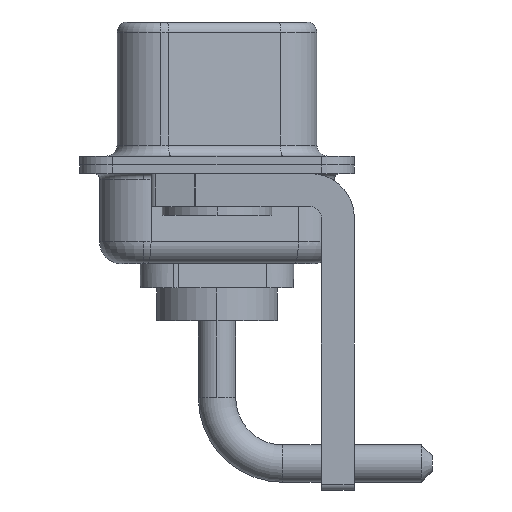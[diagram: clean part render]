
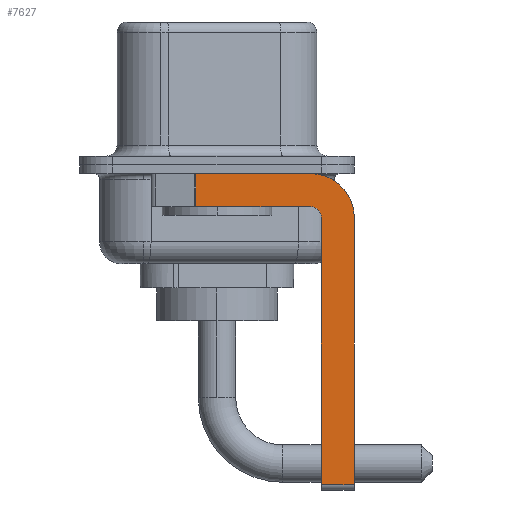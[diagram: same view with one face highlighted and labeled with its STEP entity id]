
A CAD part, left-side view. The second image highlights one B-rep face of the part: STEP entity #7627.
In plain terms, the highlighted planar face has unit normal (-1, 0, 0).
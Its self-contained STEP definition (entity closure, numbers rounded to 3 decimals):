
#83 = VECTOR ( 'NONE', #9557, 1000. ) ;
#357 = ORIENTED_EDGE ( 'NONE', *, *, #1026, .F. ) ;
#539 = VERTEX_POINT ( 'NONE', #1725 ) ;
#855 = CARTESIAN_POINT ( 'NONE',  ( -2.9, -4.25, -1.9 ) ) ;
#933 = LINE ( 'NONE', #855, #1453 ) ;
#1026 = EDGE_CURVE ( 'NONE', #9850, #12644, #933, .T. ) ;
#1371 = ORIENTED_EDGE ( 'NONE', *, *, #8969, .T. ) ;
#1448 = CARTESIAN_POINT ( 'NONE',  ( -2.9, -6.25, -2.4 ) ) ;
#1453 = VECTOR ( 'NONE', #13734, 1000. ) ;
#1725 = CARTESIAN_POINT ( 'NONE',  ( -2.9, 0.978, -0.4 ) ) ;
#1827 = DIRECTION ( 'NONE',  ( 0., -1., 0. ) ) ;
#2507 = ORIENTED_EDGE ( 'NONE', *, *, #12134, .F. ) ;
#3153 = CARTESIAN_POINT ( 'NONE',  ( -2.9, -4.25, -1.9 ) ) ;
#3434 = DIRECTION ( 'NONE',  ( 0., 0., 1. ) ) ;
#3773 = AXIS2_PLACEMENT_3D ( 'NONE', #8376, #5162, #3866 ) ;
#3866 = DIRECTION ( 'NONE',  ( 0., 0., -1. ) ) ;
#4071 = CARTESIAN_POINT ( 'NONE',  ( -2.9, -4.75, -2.4 ) ) ;
#4494 = ORIENTED_EDGE ( 'NONE', *, *, #10451, .F. ) ;
#4548 = VERTEX_POINT ( 'NONE', #13853 ) ;
#4583 = DIRECTION ( 'NONE',  ( -1., 0., 0. ) ) ;
#5088 = EDGE_CURVE ( 'NONE', #539, #12644, #9227, .T. ) ;
#5162 = DIRECTION ( 'NONE',  ( 1., 0., 0. ) ) ;
#5433 = EDGE_CURVE ( 'NONE', #11198, #10752, #10421, .T. ) ;
#5452 = CARTESIAN_POINT ( 'NONE',  ( -2.9, -4.75, -14.8 ) ) ;
#5649 = ORIENTED_EDGE ( 'NONE', *, *, #5433, .F. ) ;
#5971 = LINE ( 'NONE', #1448, #83 ) ;
#6918 = AXIS2_PLACEMENT_3D ( 'NONE', #12777, #4583, #3434 ) ;
#7002 = CARTESIAN_POINT ( 'NONE',  ( -2.9, -6.25, -2.4 ) ) ;
#7567 = PLANE ( 'NONE',  #11463 ) ;
#7627 = ADVANCED_FACE ( 'NONE', ( #12322 ), #7567, .F. ) ;
#7632 = LINE ( 'NONE', #13407, #8313 ) ;
#8090 = VECTOR ( 'NONE', #10533, 1000. ) ;
#8267 = VERTEX_POINT ( 'NONE', #7002 ) ;
#8292 = EDGE_LOOP ( 'NONE', ( #10989, #10676, #357, #4494, #5649, #1371, #12744, #2507 ) ) ;
#8313 = VECTOR ( 'NONE', #1827, 1000. ) ;
#8376 = CARTESIAN_POINT ( 'NONE',  ( -2.9, -4.25, -2.4 ) ) ;
#8795 = EDGE_CURVE ( 'NONE', #539, #11840, #7632, .T. ) ;
#8944 = CARTESIAN_POINT ( 'NONE',  ( -2.9, -4.75, -14.55 ) ) ;
#8969 = EDGE_CURVE ( 'NONE', #11198, #4548, #10297, .T. ) ;
#9178 = VECTOR ( 'NONE', #12586, 1000. ) ;
#9227 = LINE ( 'NONE', #13761, #14378 ) ;
#9557 = DIRECTION ( 'NONE',  ( 0., 0., -1. ) ) ;
#9850 = VERTEX_POINT ( 'NONE', #3153 ) ;
#10010 = DIRECTION ( 'NONE',  ( 0., 0., -1. ) ) ;
#10297 = LINE ( 'NONE', #13704, #8090 ) ;
#10360 = CIRCLE ( 'NONE', #3773, 2. ) ;
#10421 = LINE ( 'NONE', #5452, #9178 ) ;
#10451 = EDGE_CURVE ( 'NONE', #10752, #9850, #12793, .T. ) ;
#10533 = DIRECTION ( 'NONE',  ( 0., -1., 0. ) ) ;
#10676 = ORIENTED_EDGE ( 'NONE', *, *, #5088, .T. ) ;
#10752 = VERTEX_POINT ( 'NONE', #4071 ) ;
#10989 = ORIENTED_EDGE ( 'NONE', *, *, #8795, .F. ) ;
#11083 = EDGE_CURVE ( 'NONE', #8267, #4548, #5971, .T. ) ;
#11161 = CARTESIAN_POINT ( 'NONE',  ( -2.9, -4.25, -2.4 ) ) ;
#11198 = VERTEX_POINT ( 'NONE', #8944 ) ;
#11463 = AXIS2_PLACEMENT_3D ( 'NONE', #11161, #13559, #10010 ) ;
#11840 = VERTEX_POINT ( 'NONE', #15067 ) ;
#12134 = EDGE_CURVE ( 'NONE', #11840, #8267, #10360, .T. ) ;
#12322 = FACE_OUTER_BOUND ( 'NONE', #8292, .T. ) ;
#12401 = CARTESIAN_POINT ( 'NONE',  ( -2.9, 0.978, -1.9 ) ) ;
#12586 = DIRECTION ( 'NONE',  ( 0., 0., 1. ) ) ;
#12644 = VERTEX_POINT ( 'NONE', #12401 ) ;
#12744 = ORIENTED_EDGE ( 'NONE', *, *, #11083, .F. ) ;
#12777 = CARTESIAN_POINT ( 'NONE',  ( -2.9, -4.25, -2.4 ) ) ;
#12793 = CIRCLE ( 'NONE', #6918, 0.5 ) ;
#13407 = CARTESIAN_POINT ( 'NONE',  ( -2.9, 3., -0.4 ) ) ;
#13559 = DIRECTION ( 'NONE',  ( 1., 0., 0. ) ) ;
#13704 = CARTESIAN_POINT ( 'NONE',  ( -2.9, -4.25, -14.55 ) ) ;
#13734 = DIRECTION ( 'NONE',  ( 0., 1., 0. ) ) ;
#13761 = CARTESIAN_POINT ( 'NONE',  ( -2.9, 0.978, -1.9 ) ) ;
#13853 = CARTESIAN_POINT ( 'NONE',  ( -2.9, -6.25, -14.55 ) ) ;
#14378 = VECTOR ( 'NONE', #15063, 1000. ) ;
#15063 = DIRECTION ( 'NONE',  ( 0., 0., -1. ) ) ;
#15067 = CARTESIAN_POINT ( 'NONE',  ( -2.9, -4.25, -0.4 ) ) ;
